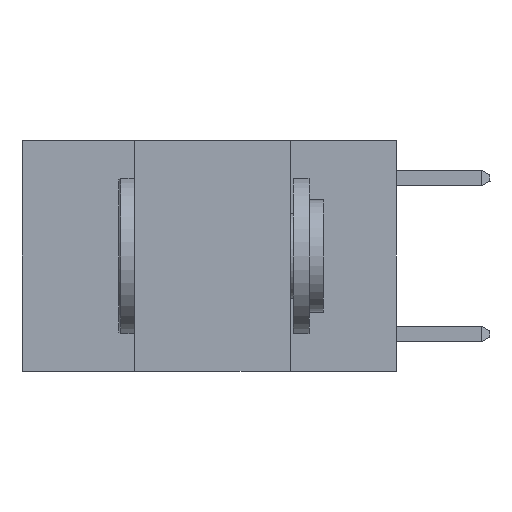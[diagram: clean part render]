
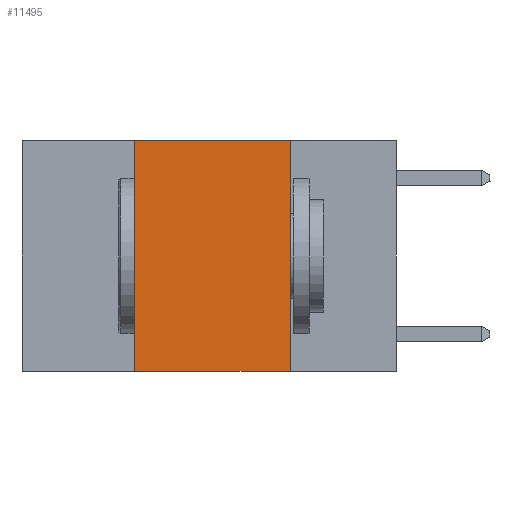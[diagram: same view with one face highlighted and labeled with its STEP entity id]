
A CAD part, left-side view. The second image highlights one B-rep face of the part: STEP entity #11495.
In plain terms, the highlighted planar face has unit normal (-1, 0, 0).
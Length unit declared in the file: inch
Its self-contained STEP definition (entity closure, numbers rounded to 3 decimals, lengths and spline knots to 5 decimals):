
#167 = ORIENTED_EDGE ( 'NONE', *, *, #3169, .F. ) ;
#1189 = VECTOR ( 'NONE', #13345, 39.37008 ) ;
#1516 = PLANE ( 'NONE',  #23438 ) ;
#1565 = VERTEX_POINT ( 'NONE', #9089 ) ;
#1803 = CARTESIAN_POINT ( 'NONE',  ( 0., 0.6, 0. ) ) ;
#2510 = ORIENTED_EDGE ( 'NONE', *, *, #6830, .F. ) ;
#3169 = EDGE_CURVE ( 'NONE', #1565, #9596, #28008, .T. ) ;
#3258 = CARTESIAN_POINT ( 'NONE',  ( 0., 0.17, 0. ) ) ;
#3527 = EDGE_CURVE ( 'NONE', #9596, #20136, #27710, .T. ) ;
#3657 = DIRECTION ( 'NONE',  ( 0., -1., 0. ) ) ;
#3783 = DIRECTION ( 'NONE',  ( 0., 0., -1. ) ) ;
#4970 = VECTOR ( 'NONE', #10772, 39.37008 ) ;
#6726 = VECTOR ( 'NONE', #25581, 39.37008 ) ;
#6830 = EDGE_CURVE ( 'NONE', #9524, #1565, #15501, .T. ) ;
#6918 = CARTESIAN_POINT ( 'NONE',  ( 0., 0.42, 0. ) ) ;
#8174 = CARTESIAN_POINT ( 'NONE',  ( 0., 0.17, 0. ) ) ;
#8351 = DIRECTION ( 'NONE',  ( 1., 0., 0. ) ) ;
#9089 = CARTESIAN_POINT ( 'NONE',  ( 0., 0.42, 0. ) ) ;
#9524 = VERTEX_POINT ( 'NONE', #19835 ) ;
#9596 = VERTEX_POINT ( 'NONE', #3258 ) ;
#10772 = DIRECTION ( 'NONE',  ( 0., -1., 0. ) ) ;
#11021 = VECTOR ( 'NONE', #3657, 39.37008 ) ;
#11495 = ADVANCED_FACE ( 'NONE', ( #18922 ), #1516, .F. ) ;
#13345 = DIRECTION ( 'NONE',  ( 0., 0., 1. ) ) ;
#13871 = CARTESIAN_POINT ( 'NONE',  ( 0., 0.17, -0.37 ) ) ;
#15501 = LINE ( 'NONE', #6918, #1189 ) ;
#15704 = LINE ( 'NONE', #23206, #11021 ) ;
#17062 = ORIENTED_EDGE ( 'NONE', *, *, #27780, .T. ) ;
#17859 = EDGE_LOOP ( 'NONE', ( #23487, #167, #2510, #17062 ) ) ;
#18922 = FACE_OUTER_BOUND ( 'NONE', #17859, .T. ) ;
#19835 = CARTESIAN_POINT ( 'NONE',  ( 0., 0.42, -0.37 ) ) ;
#20136 = VERTEX_POINT ( 'NONE', #13871 ) ;
#20676 = CARTESIAN_POINT ( 'NONE',  ( 0., 0.6, 0. ) ) ;
#23206 = CARTESIAN_POINT ( 'NONE',  ( 0., 0.6, -0.37 ) ) ;
#23438 = AXIS2_PLACEMENT_3D ( 'NONE', #1803, #8351, #3783 ) ;
#23487 = ORIENTED_EDGE ( 'NONE', *, *, #3527, .F. ) ;
#25581 = DIRECTION ( 'NONE',  ( 0., 0., -1. ) ) ;
#27710 = LINE ( 'NONE', #8174, #6726 ) ;
#27780 = EDGE_CURVE ( 'NONE', #9524, #20136, #15704, .T. ) ;
#28008 = LINE ( 'NONE', #20676, #4970 ) ;
